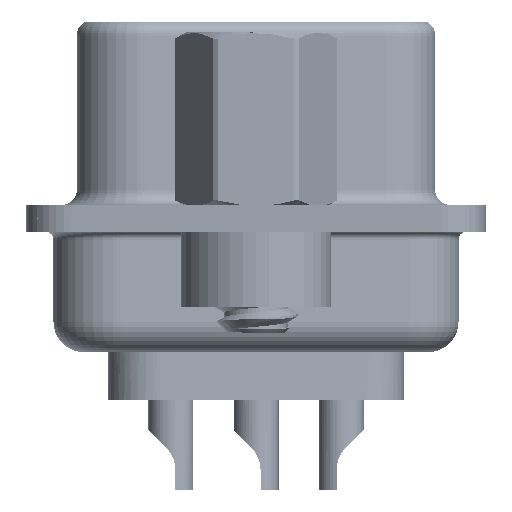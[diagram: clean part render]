
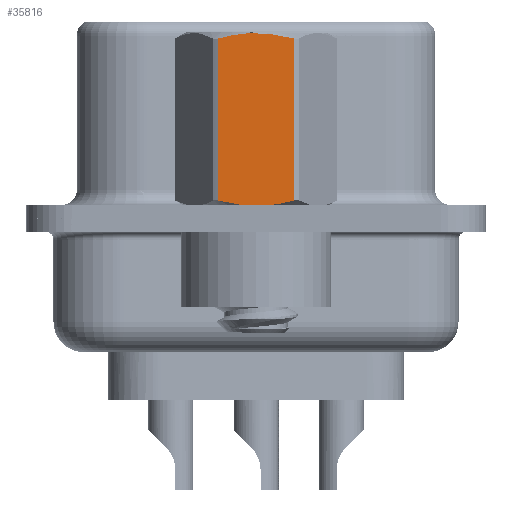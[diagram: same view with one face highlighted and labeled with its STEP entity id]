
A CAD part, left-side view. The second image highlights one B-rep face of the part: STEP entity #35816.
In plain terms, the highlighted planar face has unit normal (-1, 0, 0).
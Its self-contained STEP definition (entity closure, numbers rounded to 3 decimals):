
#321 = CARTESIAN_POINT ( 'NONE',  ( -2.381, -0.432, 6.165 ) ) ;
#696 = CARTESIAN_POINT ( 'NONE',  ( -2.381, -0.858, 6.1 ) ) ;
#1745 = CARTESIAN_POINT ( 'NONE',  ( -2.381, 1.273, 0.602 ) ) ;
#2468 = VERTEX_POINT ( 'NONE', #1745 ) ;
#2473 = DIRECTION ( 'NONE',  ( -1., 0., 0. ) ) ;
#3051 = CARTESIAN_POINT ( 'NONE',  ( -2.381, -1.273, 3.792 ) ) ;
#3608 = EDGE_LOOP ( 'NONE', ( #21731, #5606, #8015, #15748 ) ) ;
#4816 = VECTOR ( 'NONE', #20200, 1000. ) ;
#5060 = VERTEX_POINT ( 'NONE', #5455 ) ;
#5112 = CARTESIAN_POINT ( 'NONE',  ( -2.381, 1.273, 0.602 ) ) ;
#5455 = CARTESIAN_POINT ( 'NONE',  ( -2.381, -1.273, 0.602 ) ) ;
#5606 = ORIENTED_EDGE ( 'NONE', *, *, #6243, .T. ) ;
#6105 = CARTESIAN_POINT ( 'NONE',  ( -2.381, -1.273, 5.998 ) ) ;
#6243 = EDGE_CURVE ( 'NONE', #5060, #28412, #34445, .T. ) ;
#7721 = CARTESIAN_POINT ( 'NONE',  ( -2.381, -0.858, 0.5 ) ) ;
#8015 = ORIENTED_EDGE ( 'NONE', *, *, #10724, .T. ) ;
#8308 = EDGE_CURVE ( 'NONE', #11154, #2468, #31332, .T. ) ;
#8889 = CARTESIAN_POINT ( 'NONE',  ( -2.381, -0.215, 6.182 ) ) ;
#10724 = EDGE_CURVE ( 'NONE', #28412, #11154, #15089, .T. ) ;
#11154 = VERTEX_POINT ( 'NONE', #30925 ) ;
#12038 = CARTESIAN_POINT ( 'NONE',  ( -2.381, 0.428, 6.165 ) ) ;
#13283 = AXIS2_PLACEMENT_3D ( 'NONE', #22161, #2473, #22524 ) ;
#13629 = PLANE ( 'NONE',  #13283 ) ;
#14083 = CARTESIAN_POINT ( 'NONE',  ( -2.381, 1.273, 3.792 ) ) ;
#14457 = CARTESIAN_POINT ( 'NONE',  ( -2.381, -1.066, 6.054 ) ) ;
#15089 = B_SPLINE_CURVE_WITH_KNOTS ( 'NONE', 3,
 ( #6105, #14457, #696, #321, #8889, #28177, #12038, #33959, #17052, #20209 ),
 .UNSPECIFIED., .F., .F.,
 ( 4, 2, 2, 2, 4 ),
 ( 0.001, 0.002, 0.002, 0.003, 0.004 ),
 .UNSPECIFIED. ) ;
#15748 = ORIENTED_EDGE ( 'NONE', *, *, #8308, .T. ) ;
#16417 = CARTESIAN_POINT ( 'NONE',  ( -2.381, 1.065, 0.546 ) ) ;
#16611 = CARTESIAN_POINT ( 'NONE',  ( -2.381, 0.428, 0.435 ) ) ;
#17052 = CARTESIAN_POINT ( 'NONE',  ( -2.381, 1.065, 6.054 ) ) ;
#19038 = CARTESIAN_POINT ( 'NONE',  ( -2.381, -1.066, 0.546 ) ) ;
#20200 = DIRECTION ( 'NONE',  ( 0., 0., -1. ) ) ;
#20209 = CARTESIAN_POINT ( 'NONE',  ( -2.381, 1.273, 5.998 ) ) ;
#21731 = ORIENTED_EDGE ( 'NONE', *, *, #26985, .T. ) ;
#21811 = CARTESIAN_POINT ( 'NONE',  ( -2.381, 0.853, 0.499 ) ) ;
#22161 = CARTESIAN_POINT ( 'NONE',  ( -2.381, 1.375, -3.8 ) ) ;
#22524 = DIRECTION ( 'NONE',  ( 0., -1., 0. ) ) ;
#26985 = EDGE_CURVE ( 'NONE', #2468, #5060, #32262, .T. ) ;
#27546 = CARTESIAN_POINT ( 'NONE',  ( -2.381, -1.273, 0.602 ) ) ;
#27730 = CARTESIAN_POINT ( 'NONE',  ( -2.381, 0.215, 0.418 ) ) ;
#27918 = CARTESIAN_POINT ( 'NONE',  ( -2.381, -0.215, 0.418 ) ) ;
#28177 = CARTESIAN_POINT ( 'NONE',  ( -2.381, 0.215, 6.182 ) ) ;
#28412 = VERTEX_POINT ( 'NONE', #29693 ) ;
#29693 = CARTESIAN_POINT ( 'NONE',  ( -2.381, -1.273, 5.998 ) ) ;
#30925 = CARTESIAN_POINT ( 'NONE',  ( -2.381, 1.273, 5.998 ) ) ;
#31332 = LINE ( 'NONE', #14083, #4816 ) ;
#32036 = VECTOR ( 'NONE', #34075, 1000. ) ;
#32262 = B_SPLINE_CURVE_WITH_KNOTS ( 'NONE', 3,
 ( #5112, #16417, #21811, #16611, #27730, #27918, #33153, #7721, #19038, #27546 ),
 .UNSPECIFIED., .F., .F.,
 ( 4, 2, 2, 2, 4 ),
 ( 0.003, 0.003, 0.004, 0.004, 0.005 ),
 .UNSPECIFIED. ) ;
#33153 = CARTESIAN_POINT ( 'NONE',  ( -2.381, -0.432, 0.435 ) ) ;
#33959 = CARTESIAN_POINT ( 'NONE',  ( -2.381, 0.853, 6.101 ) ) ;
#34075 = DIRECTION ( 'NONE',  ( 0., 0., 1. ) ) ;
#34445 = LINE ( 'NONE', #3051, #32036 ) ;
#35816 = ADVANCED_FACE ( 'NONE', ( #36657 ), #13629, .T. ) ;
#36657 = FACE_OUTER_BOUND ( 'NONE', #3608, .T. ) ;
